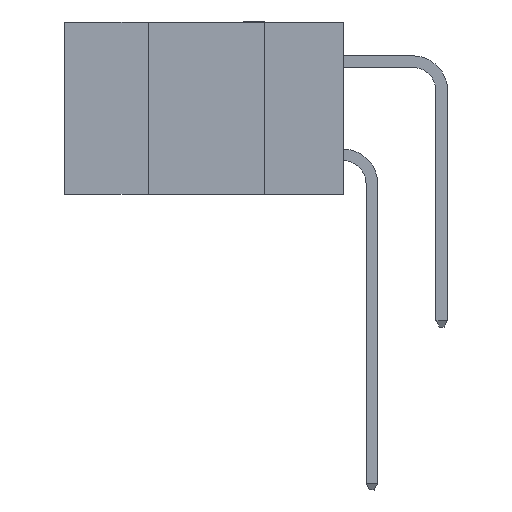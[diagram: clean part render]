
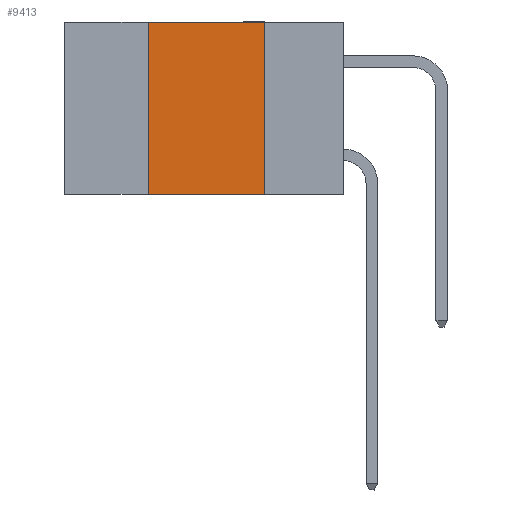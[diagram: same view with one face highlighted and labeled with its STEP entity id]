
A CAD part, left-side view. The second image highlights one B-rep face of the part: STEP entity #9413.
In plain terms, the highlighted planar face has unit normal (-1, 0, 0).
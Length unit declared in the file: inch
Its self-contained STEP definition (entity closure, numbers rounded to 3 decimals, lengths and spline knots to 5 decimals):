
#336 = ORIENTED_EDGE ( 'NONE', *, *, #5911, .F. ) ;
#428 = VERTEX_POINT ( 'NONE', #5008 ) ;
#592 = LINE ( 'NONE', #6813, #6476 ) ;
#607 = EDGE_CURVE ( 'NONE', #2968, #14102, #592, .T. ) ;
#2117 = CARTESIAN_POINT ( 'NONE',  ( 0., 0.17, -0.37 ) ) ;
#2172 = LINE ( 'NONE', #6778, #2374 ) ;
#2180 = LINE ( 'NONE', #3989, #4280 ) ;
#2374 = VECTOR ( 'NONE', #10393, 39.37008 ) ;
#2814 = LINE ( 'NONE', #7793, #8113 ) ;
#2968 = VERTEX_POINT ( 'NONE', #7418 ) ;
#3098 = EDGE_CURVE ( 'NONE', #428, #10512, #2814, .T. ) ;
#3989 = CARTESIAN_POINT ( 'NONE',  ( 0., 0.42, 0. ) ) ;
#4074 = DIRECTION ( 'NONE',  ( 1., 0., 0. ) ) ;
#4177 = ORIENTED_EDGE ( 'NONE', *, *, #3098, .T. ) ;
#4280 = VECTOR ( 'NONE', #4296, 39.37008 ) ;
#4296 = DIRECTION ( 'NONE',  ( 0., 0., 1. ) ) ;
#4723 = ORIENTED_EDGE ( 'NONE', *, *, #11674, .F. ) ;
#5008 = CARTESIAN_POINT ( 'NONE',  ( 0., 0.42, -0.37 ) ) ;
#5911 = EDGE_CURVE ( 'NONE', #428, #2968, #2180, .T. ) ;
#6113 = ORIENTED_EDGE ( 'NONE', *, *, #607, .F. ) ;
#6476 = VECTOR ( 'NONE', #7922, 39.37008 ) ;
#6561 = PLANE ( 'NONE',  #7341 ) ;
#6778 = CARTESIAN_POINT ( 'NONE',  ( 0., 0.17, 0. ) ) ;
#6813 = CARTESIAN_POINT ( 'NONE',  ( 0., 0.6, 0. ) ) ;
#7341 = AXIS2_PLACEMENT_3D ( 'NONE', #7783, #4074, #12415 ) ;
#7418 = CARTESIAN_POINT ( 'NONE',  ( 0., 0.42, 0. ) ) ;
#7783 = CARTESIAN_POINT ( 'NONE',  ( 0., 0.6, 0. ) ) ;
#7793 = CARTESIAN_POINT ( 'NONE',  ( 0., 0.6, -0.37 ) ) ;
#7922 = DIRECTION ( 'NONE',  ( 0., -1., 0. ) ) ;
#8113 = VECTOR ( 'NONE', #11257, 39.37008 ) ;
#8166 = FACE_OUTER_BOUND ( 'NONE', #12695, .T. ) ;
#9161 = CARTESIAN_POINT ( 'NONE',  ( 0., 0.17, 0. ) ) ;
#9413 = ADVANCED_FACE ( 'NONE', ( #8166 ), #6561, .F. ) ;
#10393 = DIRECTION ( 'NONE',  ( 0., 0., -1. ) ) ;
#10512 = VERTEX_POINT ( 'NONE', #2117 ) ;
#11257 = DIRECTION ( 'NONE',  ( 0., -1., 0. ) ) ;
#11674 = EDGE_CURVE ( 'NONE', #14102, #10512, #2172, .T. ) ;
#12415 = DIRECTION ( 'NONE',  ( 0., 0., -1. ) ) ;
#12695 = EDGE_LOOP ( 'NONE', ( #4723, #6113, #336, #4177 ) ) ;
#14102 = VERTEX_POINT ( 'NONE', #9161 ) ;
